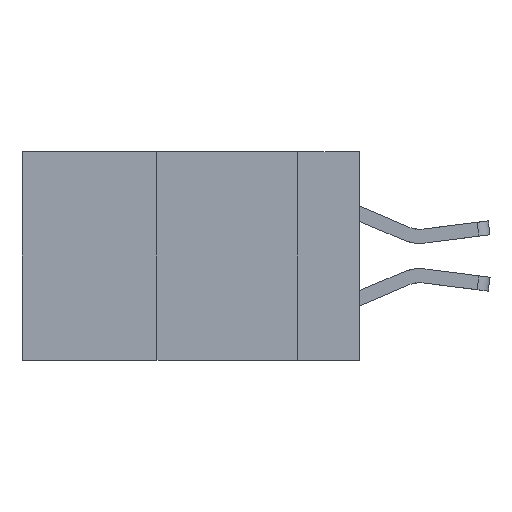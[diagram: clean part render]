
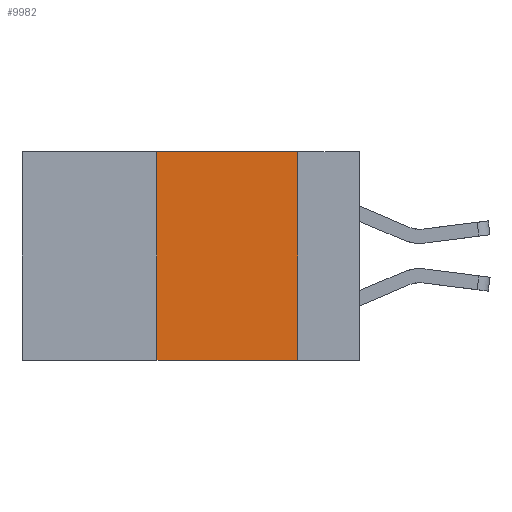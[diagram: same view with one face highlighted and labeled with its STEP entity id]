
A CAD part, left-side view. The second image highlights one B-rep face of the part: STEP entity #9982.
In plain terms, the highlighted planar face has unit normal (-1, 0, 0).
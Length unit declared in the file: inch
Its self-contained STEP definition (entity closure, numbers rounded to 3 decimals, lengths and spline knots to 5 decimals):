
#35 = DIRECTION ( 'NONE',  ( 0., 0., -1. ) ) ;
#527 = DIRECTION ( 'NONE',  ( 0., 0., -1. ) ) ;
#737 = VERTEX_POINT ( 'NONE', #4304 ) ;
#869 = VECTOR ( 'NONE', #11352, 39.37008 ) ;
#1029 = VERTEX_POINT ( 'NONE', #8516 ) ;
#1271 = VECTOR ( 'NONE', #1365, 39.37008 ) ;
#1365 = DIRECTION ( 'NONE',  ( 0., -1., 0. ) ) ;
#1888 = CARTESIAN_POINT ( 'NONE',  ( 0., 0.36, 0. ) ) ;
#2179 = VECTOR ( 'NONE', #527, 39.37008 ) ;
#2420 = LINE ( 'NONE', #6949, #1271 ) ;
#2433 = CARTESIAN_POINT ( 'NONE',  ( 0., 0.11, 0. ) ) ;
#2438 = VECTOR ( 'NONE', #2957, 39.37008 ) ;
#2910 = FACE_OUTER_BOUND ( 'NONE', #6527, .T. ) ;
#2957 = DIRECTION ( 'NONE',  ( 0., 0., 1. ) ) ;
#3472 = LINE ( 'NONE', #2433, #2179 ) ;
#4304 = CARTESIAN_POINT ( 'NONE',  ( 0., 0.11, -0.37 ) ) ;
#4407 = VERTEX_POINT ( 'NONE', #7212 ) ;
#4673 = PLANE ( 'NONE',  #7292 ) ;
#4887 = ORIENTED_EDGE ( 'NONE', *, *, #9758, .F. ) ;
#5286 = EDGE_CURVE ( 'NONE', #10726, #1029, #10279, .T. ) ;
#6433 = CARTESIAN_POINT ( 'NONE',  ( 0., 0.6, 0. ) ) ;
#6527 = EDGE_LOOP ( 'NONE', ( #4887, #10041, #11195, #6784 ) ) ;
#6771 = EDGE_CURVE ( 'NONE', #4407, #737, #2420, .T. ) ;
#6784 = ORIENTED_EDGE ( 'NONE', *, *, #6771, .T. ) ;
#6949 = CARTESIAN_POINT ( 'NONE',  ( 0., 0.6, -0.37 ) ) ;
#7212 = CARTESIAN_POINT ( 'NONE',  ( 0., 0.36, -0.37 ) ) ;
#7292 = AXIS2_PLACEMENT_3D ( 'NONE', #6433, #7456, #35 ) ;
#7456 = DIRECTION ( 'NONE',  ( 1., 0., 0. ) ) ;
#8516 = CARTESIAN_POINT ( 'NONE',  ( 0., 0.11, 0. ) ) ;
#9758 = EDGE_CURVE ( 'NONE', #1029, #737, #3472, .T. ) ;
#9982 = ADVANCED_FACE ( 'NONE', ( #2910 ), #4673, .F. ) ;
#10041 = ORIENTED_EDGE ( 'NONE', *, *, #5286, .F. ) ;
#10279 = LINE ( 'NONE', #10468, #869 ) ;
#10468 = CARTESIAN_POINT ( 'NONE',  ( 0., 0.6, 0. ) ) ;
#10470 = EDGE_CURVE ( 'NONE', #4407, #10726, #10671, .T. ) ;
#10671 = LINE ( 'NONE', #1888, #2438 ) ;
#10726 = VERTEX_POINT ( 'NONE', #11260 ) ;
#11195 = ORIENTED_EDGE ( 'NONE', *, *, #10470, .F. ) ;
#11260 = CARTESIAN_POINT ( 'NONE',  ( 0., 0.36, 0. ) ) ;
#11352 = DIRECTION ( 'NONE',  ( 0., -1., 0. ) ) ;
